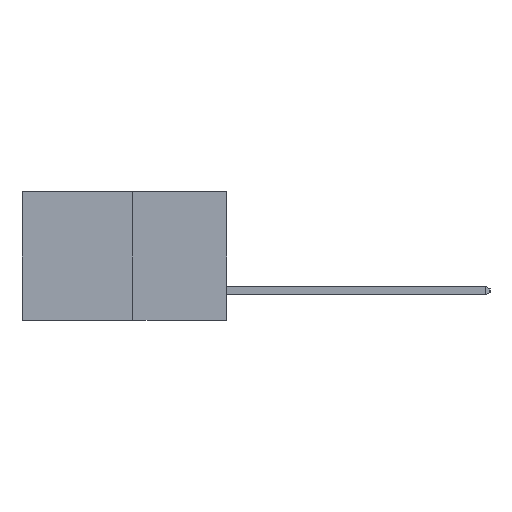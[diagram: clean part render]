
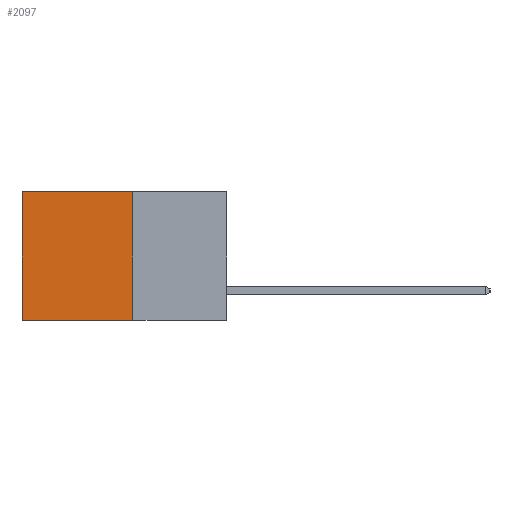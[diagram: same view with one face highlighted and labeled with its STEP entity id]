
A CAD part, left-side view. The second image highlights one B-rep face of the part: STEP entity #2097.
In plain terms, the highlighted planar face has unit normal (-1, 0, 0).
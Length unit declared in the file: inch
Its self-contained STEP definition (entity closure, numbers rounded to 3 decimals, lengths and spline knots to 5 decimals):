
#267 = VECTOR ( 'NONE', #16746, 39.37008 ) ;
#367 = ORIENTED_EDGE ( 'NONE', *, *, #15449, .F. ) ;
#1547 = VERTEX_POINT ( 'NONE', #14174 ) ;
#1569 = LINE ( 'NONE', #4845, #14841 ) ;
#2097 = ADVANCED_FACE ( 'NONE', ( #14147 ), #8285, .F. ) ;
#2471 = LINE ( 'NONE', #17542, #15173 ) ;
#2689 = VERTEX_POINT ( 'NONE', #15492 ) ;
#4465 = EDGE_CURVE ( 'NONE', #8350, #1547, #18733, .T. ) ;
#4845 = CARTESIAN_POINT ( 'NONE',  ( 0.277, 0.27, 0. ) ) ;
#5241 = EDGE_CURVE ( 'NONE', #17589, #2689, #2471, .T. ) ;
#5326 = VECTOR ( 'NONE', #12155, 39.37008 ) ;
#6843 = CARTESIAN_POINT ( 'NONE',  ( 0.277, 0.27, 0. ) ) ;
#8211 = DIRECTION ( 'NONE',  ( 0., 0., -1. ) ) ;
#8233 = DIRECTION ( 'NONE',  ( 1., 0., 0. ) ) ;
#8285 = PLANE ( 'NONE',  #18084 ) ;
#8350 = VERTEX_POINT ( 'NONE', #6843 ) ;
#10175 = ORIENTED_EDGE ( 'NONE', *, *, #19666, .T. ) ;
#11224 = CARTESIAN_POINT ( 'NONE',  ( 0.277, 0.27, -0.37 ) ) ;
#12155 = DIRECTION ( 'NONE',  ( 0., 1., 0. ) ) ;
#13944 = LINE ( 'NONE', #15685, #5326 ) ;
#14147 = FACE_OUTER_BOUND ( 'NONE', #20212, .T. ) ;
#14174 = CARTESIAN_POINT ( 'NONE',  ( 0.277, 0.27, -0.37 ) ) ;
#14841 = VECTOR ( 'NONE', #15178, 39.37008 ) ;
#15173 = VECTOR ( 'NONE', #18252, 39.37008 ) ;
#15178 = DIRECTION ( 'NONE',  ( 0., 1., 0. ) ) ;
#15449 = EDGE_CURVE ( 'NONE', #1547, #2689, #13944, .T. ) ;
#15492 = CARTESIAN_POINT ( 'NONE',  ( 0.277, 0.59, -0.37 ) ) ;
#15685 = CARTESIAN_POINT ( 'NONE',  ( 0.277, 0.27, -0.37 ) ) ;
#16318 = CARTESIAN_POINT ( 'NONE',  ( 0.277, 0.59, 0. ) ) ;
#16331 = CARTESIAN_POINT ( 'NONE',  ( 0.277, 0.27, -0.37 ) ) ;
#16502 = ORIENTED_EDGE ( 'NONE', *, *, #5241, .T. ) ;
#16746 = DIRECTION ( 'NONE',  ( 0., 0., -1. ) ) ;
#17542 = CARTESIAN_POINT ( 'NONE',  ( 0.277, 0.59, -0.37 ) ) ;
#17589 = VERTEX_POINT ( 'NONE', #16318 ) ;
#18084 = AXIS2_PLACEMENT_3D ( 'NONE', #11224, #8233, #8211 ) ;
#18252 = DIRECTION ( 'NONE',  ( 0., 0., -1. ) ) ;
#18733 = LINE ( 'NONE', #16331, #267 ) ;
#19666 = EDGE_CURVE ( 'NONE', #8350, #17589, #1569, .T. ) ;
#19809 = ORIENTED_EDGE ( 'NONE', *, *, #4465, .F. ) ;
#20212 = EDGE_LOOP ( 'NONE', ( #16502, #367, #19809, #10175 ) ) ;
